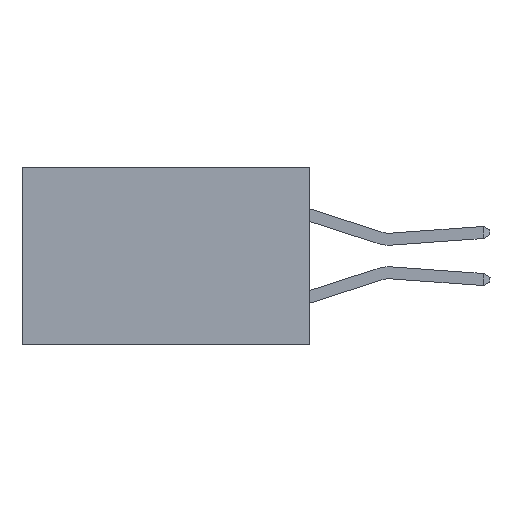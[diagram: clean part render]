
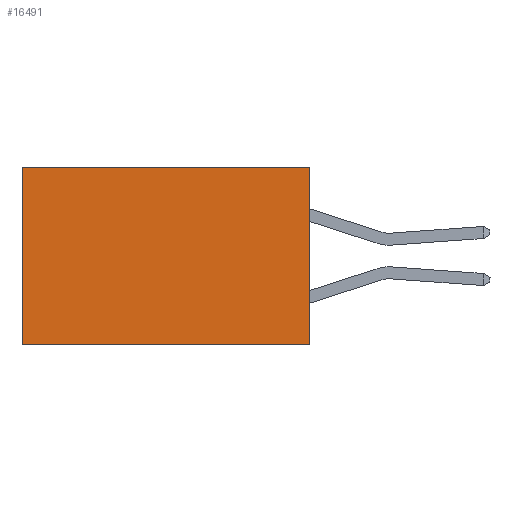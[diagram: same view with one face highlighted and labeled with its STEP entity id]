
A CAD part, left-side view. The second image highlights one B-rep face of the part: STEP entity #16491.
In plain terms, the highlighted planar face has unit normal (-1, 0, 0).
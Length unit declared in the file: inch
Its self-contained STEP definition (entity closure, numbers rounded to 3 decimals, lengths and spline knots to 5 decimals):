
#144 = ORIENTED_EDGE ( 'NONE', *, *, #19925, .F. ) ;
#334 = CARTESIAN_POINT ( 'NONE',  ( 0.298, 0., 0. ) ) ;
#838 = DIRECTION ( 'NONE',  ( 0., 0., -1. ) ) ;
#1450 = PLANE ( 'NONE',  #5222 ) ;
#1885 = ORIENTED_EDGE ( 'NONE', *, *, #23020, .F. ) ;
#2586 = VECTOR ( 'NONE', #838, 39.37008 ) ;
#3138 = VERTEX_POINT ( 'NONE', #334 ) ;
#3654 = DIRECTION ( 'NONE',  ( 1., 0., 0. ) ) ;
#3969 = ORIENTED_EDGE ( 'NONE', *, *, #4319, .T. ) ;
#4319 = EDGE_CURVE ( 'NONE', #27038, #8673, #25999, .T. ) ;
#4707 = LINE ( 'NONE', #16460, #25625 ) ;
#5222 = AXIS2_PLACEMENT_3D ( 'NONE', #16298, #3654, #18406 ) ;
#6085 = ORIENTED_EDGE ( 'NONE', *, *, #23998, .T. ) ;
#8295 = DIRECTION ( 'NONE',  ( 0., 1., 0. ) ) ;
#8673 = VERTEX_POINT ( 'NONE', #22302 ) ;
#11498 = CARTESIAN_POINT ( 'NONE',  ( 0.298, 0.6, 0. ) ) ;
#12493 = VECTOR ( 'NONE', #8295, 39.37008 ) ;
#13588 = CARTESIAN_POINT ( 'NONE',  ( 0.298, 0., 0. ) ) ;
#14063 = VERTEX_POINT ( 'NONE', #20904 ) ;
#14653 = CARTESIAN_POINT ( 'NONE',  ( 0.298, 0., 0. ) ) ;
#16298 = CARTESIAN_POINT ( 'NONE',  ( 0.298, 0., 0. ) ) ;
#16460 = CARTESIAN_POINT ( 'NONE',  ( 0.298, 0., -0.37 ) ) ;
#16491 = ADVANCED_FACE ( 'NONE', ( #23300 ), #1450, .F. ) ;
#17417 = LINE ( 'NONE', #14653, #12493 ) ;
#18406 = DIRECTION ( 'NONE',  ( 0., 0., -1. ) ) ;
#18475 = DIRECTION ( 'NONE',  ( 0., 1., 0. ) ) ;
#19925 = EDGE_CURVE ( 'NONE', #14063, #8673, #4707, .T. ) ;
#20904 = CARTESIAN_POINT ( 'NONE',  ( 0.298, 0., -0.37 ) ) ;
#22302 = CARTESIAN_POINT ( 'NONE',  ( 0.298, 0.6, -0.37 ) ) ;
#23020 = EDGE_CURVE ( 'NONE', #3138, #14063, #24299, .T. ) ;
#23300 = FACE_OUTER_BOUND ( 'NONE', #26570, .T. ) ;
#23998 = EDGE_CURVE ( 'NONE', #3138, #27038, #17417, .T. ) ;
#24299 = LINE ( 'NONE', #13588, #2586 ) ;
#25599 = DIRECTION ( 'NONE',  ( 0., 0., -1. ) ) ;
#25625 = VECTOR ( 'NONE', #18475, 39.37008 ) ;
#25999 = LINE ( 'NONE', #11498, #26643 ) ;
#26320 = CARTESIAN_POINT ( 'NONE',  ( 0.298, 0.6, 0. ) ) ;
#26570 = EDGE_LOOP ( 'NONE', ( #3969, #144, #1885, #6085 ) ) ;
#26643 = VECTOR ( 'NONE', #25599, 39.37008 ) ;
#27038 = VERTEX_POINT ( 'NONE', #26320 ) ;
